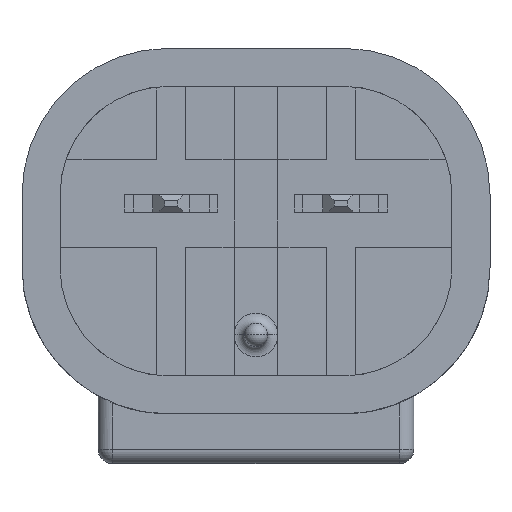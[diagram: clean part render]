
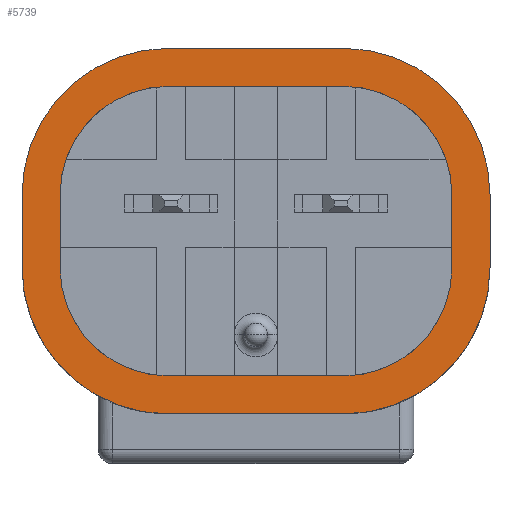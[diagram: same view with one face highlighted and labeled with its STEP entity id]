
A CAD part, front view. The second image highlights one B-rep face of the part: STEP entity #5739.
In plain terms, the highlighted planar face has unit normal (0, -1, 0).
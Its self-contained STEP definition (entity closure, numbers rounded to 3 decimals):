
#54 = ORIENTED_EDGE ( 'NONE', *, *, #2906, .F. ) ;
#75 = ORIENTED_EDGE ( 'NONE', *, *, #4999, .F. ) ;
#193 = CARTESIAN_POINT ( 'NONE',  ( -3., 0., -7.5 ) ) ;
#214 = CIRCLE ( 'NONE', #1997, 5. ) ;
#219 = FACE_BOUND ( 'NONE', #2569, .T. ) ;
#227 = DIRECTION ( 'NONE',  ( 1., 0., 0. ) ) ;
#232 = VERTEX_POINT ( 'NONE', #4660 ) ;
#252 = CARTESIAN_POINT ( 'NONE',  ( -3., 0., -11.2 ) ) ;
#297 = CARTESIAN_POINT ( 'NONE',  ( -3., 0., -12.5 ) ) ;
#327 = CARTESIAN_POINT ( 'NONE',  ( 6.7, 0., -7.5 ) ) ;
#341 = LINE ( 'NONE', #841, #1823 ) ;
#372 = VERTEX_POINT ( 'NONE', #3480 ) ;
#437 = EDGE_CURVE ( 'NONE', #1376, #232, #1746, .T. ) ;
#513 = ORIENTED_EDGE ( 'NONE', *, *, #437, .F. ) ;
#579 = EDGE_CURVE ( 'NONE', #1895, #4411, #3349, .T. ) ;
#611 = CARTESIAN_POINT ( 'NONE',  ( 3., 0., -7.5 ) ) ;
#619 = CARTESIAN_POINT ( 'NONE',  ( 6.7, 0., -6.8 ) ) ;
#642 = VECTOR ( 'NONE', #2696, 1000. ) ;
#657 = ORIENTED_EDGE ( 'NONE', *, *, #4115, .F. ) ;
#697 = DIRECTION ( 'NONE',  ( 0., -1., 0. ) ) ;
#740 = ORIENTED_EDGE ( 'NONE', *, *, #2800, .F. ) ;
#805 = VERTEX_POINT ( 'NONE', #4393 ) ;
#819 = FACE_OUTER_BOUND ( 'NONE', #2205, .T. ) ;
#823 = CARTESIAN_POINT ( 'NONE',  ( 3., 0., -12.5 ) ) ;
#841 = CARTESIAN_POINT ( 'NONE',  ( -3., 0., -12.5 ) ) ;
#1149 = EDGE_CURVE ( 'NONE', #5588, #1376, #2966, .T. ) ;
#1153 = AXIS2_PLACEMENT_3D ( 'NONE', #1544, #2890, #4693 ) ;
#1169 = DIRECTION ( 'NONE',  ( 0., 1., 0. ) ) ;
#1183 = EDGE_CURVE ( 'NONE', #2015, #1663, #1230, .T. ) ;
#1199 = CARTESIAN_POINT ( 'NONE',  ( -3., 0., 0. ) ) ;
#1208 = CARTESIAN_POINT ( 'NONE',  ( -8., 0., -7.5 ) ) ;
#1222 = AXIS2_PLACEMENT_3D ( 'NONE', #4671, #697, #1580 ) ;
#1230 = LINE ( 'NONE', #1199, #2023 ) ;
#1286 = VERTEX_POINT ( 'NONE', #1398 ) ;
#1293 = AXIS2_PLACEMENT_3D ( 'NONE', #2335, #5004, #3634 ) ;
#1374 = CARTESIAN_POINT ( 'NONE',  ( -6.7, 0., -7.5 ) ) ;
#1376 = VERTEX_POINT ( 'NONE', #3387 ) ;
#1398 = CARTESIAN_POINT ( 'NONE',  ( 8., 0., -7.5 ) ) ;
#1444 = CARTESIAN_POINT ( 'NONE',  ( 3., 0., 0. ) ) ;
#1502 = DIRECTION ( 'NONE',  ( 0., 1., 0. ) ) ;
#1544 = CARTESIAN_POINT ( 'NONE',  ( 3., 0., -7.5 ) ) ;
#1580 = DIRECTION ( 'NONE',  ( 1., 0., 0. ) ) ;
#1647 = ORIENTED_EDGE ( 'NONE', *, *, #579, .F. ) ;
#1663 = VERTEX_POINT ( 'NONE', #1444 ) ;
#1727 = CIRCLE ( 'NONE', #1153, 3.7 ) ;
#1743 = CIRCLE ( 'NONE', #4746, 5. ) ;
#1746 = LINE ( 'NONE', #1208, #5327 ) ;
#1823 = VECTOR ( 'NONE', #2135, 1000. ) ;
#1849 = CARTESIAN_POINT ( 'NONE',  ( -6.7, 0., -6.8 ) ) ;
#1895 = VERTEX_POINT ( 'NONE', #327 ) ;
#1898 = LINE ( 'NONE', #5420, #2956 ) ;
#1913 = VERTEX_POINT ( 'NONE', #3146 ) ;
#1950 = ORIENTED_EDGE ( 'NONE', *, *, #1149, .F. ) ;
#1997 = AXIS2_PLACEMENT_3D ( 'NONE', #2912, #1502, #2473 ) ;
#2015 = VERTEX_POINT ( 'NONE', #4063 ) ;
#2023 = VECTOR ( 'NONE', #227, 1000. ) ;
#2027 = ORIENTED_EDGE ( 'NONE', *, *, #3092, .F. ) ;
#2038 = ORIENTED_EDGE ( 'NONE', *, *, #5382, .F. ) ;
#2079 = ORIENTED_EDGE ( 'NONE', *, *, #1183, .F. ) ;
#2108 = DIRECTION ( 'NONE',  ( -1., 0., 0. ) ) ;
#2135 = DIRECTION ( 'NONE',  ( -1., 0., 0. ) ) ;
#2192 = AXIS2_PLACEMENT_3D ( 'NONE', #193, #3310, #5100 ) ;
#2205 = EDGE_LOOP ( 'NONE', ( #5006, #2079, #54, #513, #1950, #4275, #2489, #740 ) ) ;
#2329 = CIRCLE ( 'NONE', #1293, 3.7 ) ;
#2335 = CARTESIAN_POINT ( 'NONE',  ( 3., 0., -5. ) ) ;
#2353 = EDGE_CURVE ( 'NONE', #372, #5061, #3668, .T. ) ;
#2473 = DIRECTION ( 'NONE',  ( -1., 0., 0. ) ) ;
#2489 = ORIENTED_EDGE ( 'NONE', *, *, #4716, .F. ) ;
#2495 = AXIS2_PLACEMENT_3D ( 'NONE', #5711, #2512, #2108 ) ;
#2512 = DIRECTION ( 'NONE',  ( 0., -1., 0. ) ) ;
#2537 = CIRCLE ( 'NONE', #1222, 3.7 ) ;
#2569 = EDGE_LOOP ( 'NONE', ( #2038, #1647, #2027, #3442, #657, #3191, #4027, #75 ) ) ;
#2687 = LINE ( 'NONE', #4104, #4080 ) ;
#2696 = DIRECTION ( 'NONE',  ( 0., 0., -1. ) ) ;
#2719 = DIRECTION ( 'NONE',  ( -1., 0., 0. ) ) ;
#2721 = CARTESIAN_POINT ( 'NONE',  ( -3., 0., -5. ) ) ;
#2785 = CARTESIAN_POINT ( 'NONE',  ( 8., 0., -5. ) ) ;
#2800 = EDGE_CURVE ( 'NONE', #3946, #1286, #1898, .T. ) ;
#2869 = DIRECTION ( 'NONE',  ( 1., 0., 0. ) ) ;
#2890 = DIRECTION ( 'NONE',  ( 0., -1., 0. ) ) ;
#2906 = EDGE_CURVE ( 'NONE', #232, #2015, #1743, .T. ) ;
#2912 = CARTESIAN_POINT ( 'NONE',  ( 3., 0., -5. ) ) ;
#2923 = PLANE ( 'NONE',  #2495 ) ;
#2956 = VECTOR ( 'NONE', #3696, 1000. ) ;
#2966 = CIRCLE ( 'NONE', #4277, 5. ) ;
#3092 = EDGE_CURVE ( 'NONE', #805, #1895, #1727, .T. ) ;
#3100 = AXIS2_PLACEMENT_3D ( 'NONE', #611, #4281, #2869 ) ;
#3146 = CARTESIAN_POINT ( 'NONE',  ( -3., 0., -1.3 ) ) ;
#3191 = ORIENTED_EDGE ( 'NONE', *, *, #2353, .F. ) ;
#3207 = EDGE_CURVE ( 'NONE', #4885, #5588, #341, .T. ) ;
#3261 = EDGE_CURVE ( 'NONE', #4755, #805, #2687, .T. ) ;
#3310 = DIRECTION ( 'NONE',  ( 0., -1., 0. ) ) ;
#3341 = EDGE_CURVE ( 'NONE', #1663, #3946, #214, .T. ) ;
#3349 = LINE ( 'NONE', #619, #3476 ) ;
#3387 = CARTESIAN_POINT ( 'NONE',  ( -8., 0., -7.5 ) ) ;
#3442 = ORIENTED_EDGE ( 'NONE', *, *, #3261, .F. ) ;
#3476 = VECTOR ( 'NONE', #5602, 1000. ) ;
#3480 = CARTESIAN_POINT ( 'NONE',  ( -6.7, 0., -5. ) ) ;
#3580 = DIRECTION ( 'NONE',  ( 1., 0., 0. ) ) ;
#3634 = DIRECTION ( 'NONE',  ( -1., 0., 0. ) ) ;
#3641 = LINE ( 'NONE', #5013, #4982 ) ;
#3668 = LINE ( 'NONE', #1849, #642 ) ;
#3675 = VERTEX_POINT ( 'NONE', #3766 ) ;
#3696 = DIRECTION ( 'NONE',  ( 0., 0., -1. ) ) ;
#3724 = DIRECTION ( 'NONE',  ( 0., 1., 0. ) ) ;
#3766 = CARTESIAN_POINT ( 'NONE',  ( 3., 0., -1.3 ) ) ;
#3825 = CARTESIAN_POINT ( 'NONE',  ( -3., 0., -7.5 ) ) ;
#3946 = VERTEX_POINT ( 'NONE', #2785 ) ;
#3959 = CIRCLE ( 'NONE', #3100, 5. ) ;
#4027 = ORIENTED_EDGE ( 'NONE', *, *, #4749, .F. ) ;
#4063 = CARTESIAN_POINT ( 'NONE',  ( -3., 0., 0. ) ) ;
#4080 = VECTOR ( 'NONE', #4153, 1000. ) ;
#4104 = CARTESIAN_POINT ( 'NONE',  ( 2.4, 0., -11.2 ) ) ;
#4115 = EDGE_CURVE ( 'NONE', #5061, #4755, #4725, .T. ) ;
#4153 = DIRECTION ( 'NONE',  ( 1., 0., 0. ) ) ;
#4163 = DIRECTION ( 'NONE',  ( 1., 0., 0. ) ) ;
#4275 = ORIENTED_EDGE ( 'NONE', *, *, #3207, .F. ) ;
#4277 = AXIS2_PLACEMENT_3D ( 'NONE', #3825, #1169, #3580 ) ;
#4281 = DIRECTION ( 'NONE',  ( 0., 1., 0. ) ) ;
#4393 = CARTESIAN_POINT ( 'NONE',  ( 3., 0., -11.2 ) ) ;
#4411 = VERTEX_POINT ( 'NONE', #4549 ) ;
#4549 = CARTESIAN_POINT ( 'NONE',  ( 6.7, 0., -5. ) ) ;
#4660 = CARTESIAN_POINT ( 'NONE',  ( -8., 0., -5. ) ) ;
#4671 = CARTESIAN_POINT ( 'NONE',  ( -3., 0., -5. ) ) ;
#4693 = DIRECTION ( 'NONE',  ( -1., 0., 0. ) ) ;
#4716 = EDGE_CURVE ( 'NONE', #1286, #4885, #3959, .T. ) ;
#4725 = CIRCLE ( 'NONE', #2192, 3.7 ) ;
#4746 = AXIS2_PLACEMENT_3D ( 'NONE', #2721, #3724, #4163 ) ;
#4749 = EDGE_CURVE ( 'NONE', #1913, #372, #2537, .T. ) ;
#4755 = VERTEX_POINT ( 'NONE', #252 ) ;
#4841 = DIRECTION ( 'NONE',  ( 0., 0., 1. ) ) ;
#4885 = VERTEX_POINT ( 'NONE', #823 ) ;
#4982 = VECTOR ( 'NONE', #2719, 1000. ) ;
#4999 = EDGE_CURVE ( 'NONE', #3675, #1913, #3641, .T. ) ;
#5004 = DIRECTION ( 'NONE',  ( 0., -1., 0. ) ) ;
#5006 = ORIENTED_EDGE ( 'NONE', *, *, #3341, .F. ) ;
#5013 = CARTESIAN_POINT ( 'NONE',  ( 0.75, 0., -1.3 ) ) ;
#5061 = VERTEX_POINT ( 'NONE', #1374 ) ;
#5100 = DIRECTION ( 'NONE',  ( 1., 0., 0. ) ) ;
#5327 = VECTOR ( 'NONE', #4841, 1000. ) ;
#5382 = EDGE_CURVE ( 'NONE', #4411, #3675, #2329, .T. ) ;
#5420 = CARTESIAN_POINT ( 'NONE',  ( 8., 0., -7.5 ) ) ;
#5588 = VERTEX_POINT ( 'NONE', #297 ) ;
#5602 = DIRECTION ( 'NONE',  ( 0., 0., 1. ) ) ;
#5711 = CARTESIAN_POINT ( 'NONE',  ( 3., 0., -5. ) ) ;
#5739 = ADVANCED_FACE ( 'NONE', ( #219, #819 ), #2923, .T. ) ;
